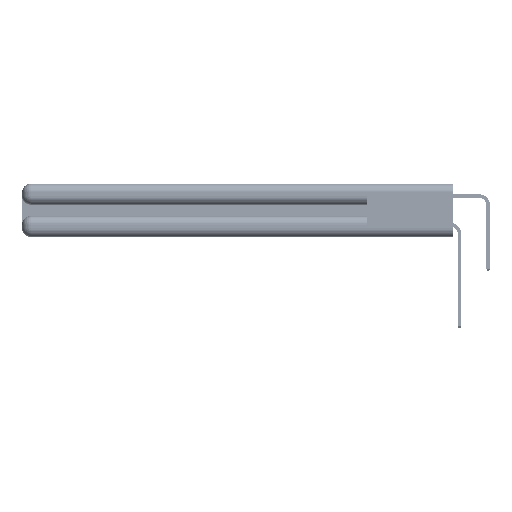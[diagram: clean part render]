
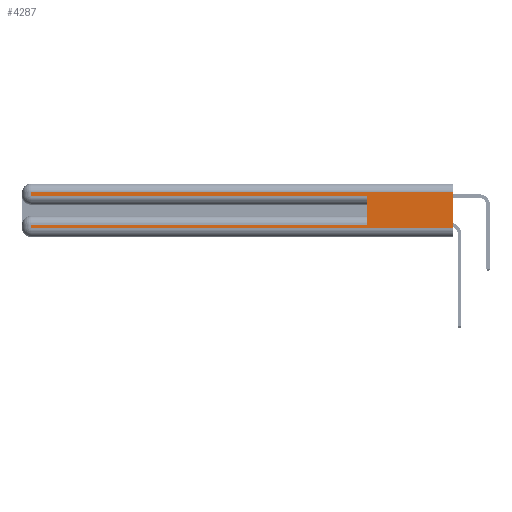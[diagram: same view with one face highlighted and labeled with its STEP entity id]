
A CAD part, left-side view. The second image highlights one B-rep face of the part: STEP entity #4287.
In plain terms, the highlighted planar face has unit normal (-1, 0, 0).
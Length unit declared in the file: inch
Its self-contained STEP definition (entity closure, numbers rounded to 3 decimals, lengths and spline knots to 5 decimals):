
#1232 = DIRECTION ( 'NONE',  ( 0., 0., -1. ) ) ;
#1784 = EDGE_CURVE ( 'NONE', #4165, #44158, #32121, .T. ) ;
#2333 = CARTESIAN_POINT ( 'NONE',  ( 0., 2.94, 0.285 ) ) ;
#2407 = VERTEX_POINT ( 'NONE', #39997 ) ;
#2669 = CARTESIAN_POINT ( 'NONE',  ( 0., 0., 0.31 ) ) ;
#3190 = EDGE_CURVE ( 'NONE', #44497, #19273, #51407, .T. ) ;
#3711 = DIRECTION ( 'NONE',  ( 0., 1., 0. ) ) ;
#4165 = VERTEX_POINT ( 'NONE', #2333 ) ;
#4287 = ADVANCED_FACE ( 'NONE', ( #25081 ), #51113, .F. ) ;
#6260 = VERTEX_POINT ( 'NONE', #23421 ) ;
#6780 = CARTESIAN_POINT ( 'NONE',  ( 0., 0.6, 0.285 ) ) ;
#7027 = DIRECTION ( 'NONE',  ( 1., 0., 0. ) ) ;
#7298 = VERTEX_POINT ( 'NONE', #33280 ) ;
#10541 = DIRECTION ( 'NONE',  ( 0., 0., 1. ) ) ;
#11328 = DIRECTION ( 'NONE',  ( 0., -1., 0. ) ) ;
#12991 = CARTESIAN_POINT ( 'NONE',  ( 0., 2.94, 0.06 ) ) ;
#13581 = VECTOR ( 'NONE', #23008, 39.37008 ) ;
#13731 = EDGE_CURVE ( 'NONE', #6260, #27185, #45664, .T. ) ;
#17420 = CARTESIAN_POINT ( 'NONE',  ( 0., 2.94, 0.31 ) ) ;
#18094 = ORIENTED_EDGE ( 'NONE', *, *, #41718, .F. ) ;
#18147 = ORIENTED_EDGE ( 'NONE', *, *, #13731, .T. ) ;
#18907 = ORIENTED_EDGE ( 'NONE', *, *, #32678, .T. ) ;
#19008 = ORIENTED_EDGE ( 'NONE', *, *, #1784, .T. ) ;
#19273 = VERTEX_POINT ( 'NONE', #27538 ) ;
#19498 = VECTOR ( 'NONE', #33248, 39.37008 ) ;
#19690 = ORIENTED_EDGE ( 'NONE', *, *, #44081, .F. ) ;
#19836 = ORIENTED_EDGE ( 'NONE', *, *, #21627, .T. ) ;
#20397 = ORIENTED_EDGE ( 'NONE', *, *, #37733, .T. ) ;
#21627 = EDGE_CURVE ( 'NONE', #2407, #7298, #32029, .T. ) ;
#22309 = VECTOR ( 'NONE', #43852, 39.37008 ) ;
#23008 = DIRECTION ( 'NONE',  ( 0., 1., 0. ) ) ;
#23421 = CARTESIAN_POINT ( 'NONE',  ( 0., 0., 0.31 ) ) ;
#24376 = VECTOR ( 'NONE', #37247, 39.37008 ) ;
#25081 = FACE_OUTER_BOUND ( 'NONE', #36857, .T. ) ;
#25610 = CARTESIAN_POINT ( 'NONE',  ( 0., 2.94, 0.37 ) ) ;
#25632 = LINE ( 'NONE', #33213, #24376 ) ;
#27185 = VERTEX_POINT ( 'NONE', #17420 ) ;
#27538 = CARTESIAN_POINT ( 'NONE',  ( 0., 0., 0.06 ) ) ;
#28711 = AXIS2_PLACEMENT_3D ( 'NONE', #31277, #7027, #35305 ) ;
#30592 = VECTOR ( 'NONE', #10541, 39.37008 ) ;
#30793 = VECTOR ( 'NONE', #3711, 39.37008 ) ;
#30883 = VECTOR ( 'NONE', #11328, 39.37008 ) ;
#31277 = CARTESIAN_POINT ( 'NONE',  ( 0., 0., 0.37 ) ) ;
#32029 = LINE ( 'NONE', #51940, #30793 ) ;
#32121 = LINE ( 'NONE', #39506, #30883 ) ;
#32678 = EDGE_CURVE ( 'NONE', #27185, #4165, #44138, .T. ) ;
#33213 = CARTESIAN_POINT ( 'NONE',  ( 0., 0., 0.37 ) ) ;
#33248 = DIRECTION ( 'NONE',  ( 0., -1., 0. ) ) ;
#33280 = CARTESIAN_POINT ( 'NONE',  ( 0., 2.94, 0.085 ) ) ;
#35305 = DIRECTION ( 'NONE',  ( 0., 0., -1. ) ) ;
#36857 = EDGE_LOOP ( 'NONE', ( #18094, #18147, #18907, #19008, #19690, #19836, #20397, #51280 ) ) ;
#37247 = DIRECTION ( 'NONE',  ( 0., 0., -1. ) ) ;
#37733 = EDGE_CURVE ( 'NONE', #7298, #44497, #48459, .T. ) ;
#38568 = CARTESIAN_POINT ( 'NONE',  ( 0., 0.6, 0.145 ) ) ;
#39099 = VECTOR ( 'NONE', #1232, 39.37008 ) ;
#39506 = CARTESIAN_POINT ( 'NONE',  ( 0., 0., 0.285 ) ) ;
#39871 = CARTESIAN_POINT ( 'NONE',  ( 0., 2.94, 0.37 ) ) ;
#39997 = CARTESIAN_POINT ( 'NONE',  ( 0., 0.6, 0.085 ) ) ;
#41718 = EDGE_CURVE ( 'NONE', #6260, #19273, #25632, .T. ) ;
#42454 = LINE ( 'NONE', #38568, #30592 ) ;
#43852 = DIRECTION ( 'NONE',  ( 0., 0., -1. ) ) ;
#44081 = EDGE_CURVE ( 'NONE', #2407, #44158, #42454, .T. ) ;
#44138 = LINE ( 'NONE', #39871, #22309 ) ;
#44158 = VERTEX_POINT ( 'NONE', #6780 ) ;
#44497 = VERTEX_POINT ( 'NONE', #12991 ) ;
#45664 = LINE ( 'NONE', #2669, #13581 ) ;
#48459 = LINE ( 'NONE', #25610, #39099 ) ;
#48960 = CARTESIAN_POINT ( 'NONE',  ( 0., 0., 0.06 ) ) ;
#51113 = PLANE ( 'NONE',  #28711 ) ;
#51280 = ORIENTED_EDGE ( 'NONE', *, *, #3190, .T. ) ;
#51407 = LINE ( 'NONE', #48960, #19498 ) ;
#51940 = CARTESIAN_POINT ( 'NONE',  ( 0., 0., 0.085 ) ) ;
